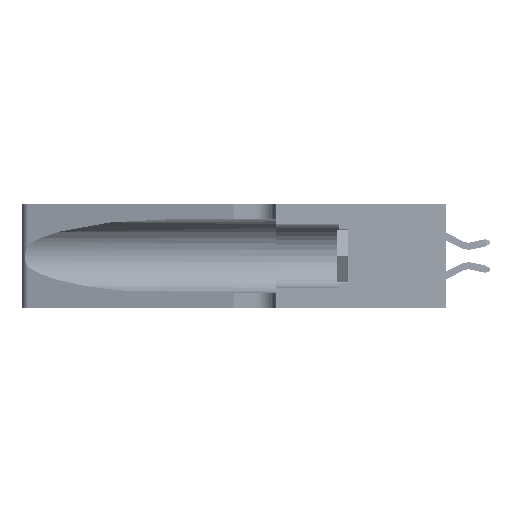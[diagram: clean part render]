
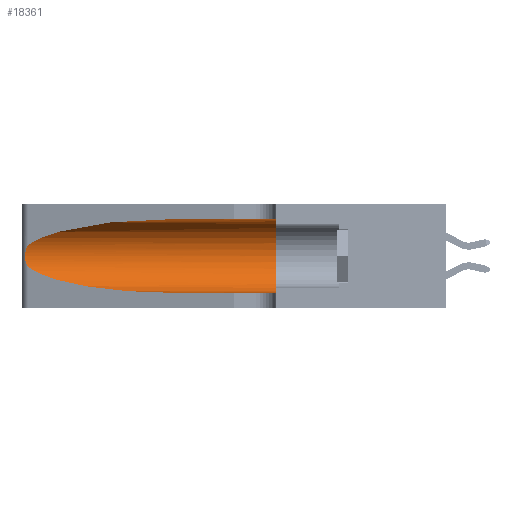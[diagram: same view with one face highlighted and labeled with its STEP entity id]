
A CAD part, left-side view. The second image highlights one B-rep face of the part: STEP entity #18361.
In plain terms, the highlighted cylindrical face has radius 3.308 mm (diameter 6.617 mm), a partial arc.
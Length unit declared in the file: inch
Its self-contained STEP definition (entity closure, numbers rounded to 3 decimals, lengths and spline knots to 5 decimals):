
#403 = ORIENTED_EDGE ( 'NONE', *, *, #45764, .T. ) ;
#1834 = CARTESIAN_POINT ( 'NONE',  ( 0.1305, 0.35, 0.05475 ) ) ;
#2414 = CARTESIAN_POINT ( 'NONE',  ( 0.25787, 1.23484, 0.2124 ) ) ;
#2507 = VERTEX_POINT ( 'NONE', #43651 ) ;
#5324 = FACE_OUTER_BOUND ( 'NONE', #14795, .T. ) ;
#5396 =( BOUNDED_CURVE ( )  B_SPLINE_CURVE ( 3, ( #17493, #8885, #21768, #51166 ),
 .UNSPECIFIED., .F., .F. ) 
 B_SPLINE_CURVE_WITH_KNOTS ( ( 4, 4 ),
 ( 3.44316, 4.71239 ),
 .UNSPECIFIED. ) 
 CURVE ( )  GEOMETRIC_REPRESENTATION_ITEM ( )  RATIONAL_B_SPLINE_CURVE ( ( 1., 0.87, 0.87, 1. ) ) 
 REPRESENTATION_ITEM ( '' )  );
#6060 = DIRECTION ( 'NONE',  ( 0., -1., 0. ) ) ;
#6214 = DIRECTION ( 'NONE',  ( 0., -1., 0. ) ) ;
#6706 = CARTESIAN_POINT ( 'NONE',  ( 0.26018, 1.23835, 0.19895 ) ) ;
#8131 = VERTEX_POINT ( 'NONE', #1834 ) ;
#8208 = EDGE_CURVE ( 'NONE', #21426, #42346, #44751, .T. ) ;
#8885 = CARTESIAN_POINT ( 'NONE',  ( 0.2373, 1.15595, 0.08982 ) ) ;
#11034 = CARTESIAN_POINT ( 'NONE',  ( 0.26075, 1.23896, 0.178 ) ) ;
#13370 = ORIENTED_EDGE ( 'NONE', *, *, #25348, .T. ) ;
#13740 = CARTESIAN_POINT ( 'NONE',  ( 0.1305, 0.35, 0.185 ) ) ;
#13960 = DIRECTION ( 'NONE',  ( 0., 0., -1. ) ) ;
#14795 = EDGE_LOOP ( 'NONE', ( #403, #54243, #37946, #13370, #43598, #37337 ) ) ;
#15139 = CARTESIAN_POINT ( 'NONE',  ( 0.25639, 1.23184, 0.21858 ) ) ;
#15327 = CARTESIAN_POINT ( 'NONE',  ( 0.25856, 1.23593, 0.16098 ) ) ;
#15800 = CARTESIAN_POINT ( 'NONE',  ( 0.1305, 0.72297, 0.05475 ) ) ;
#16131 = VECTOR ( 'NONE', #6060, 39.37008 ) ;
#16609 = CYLINDRICAL_SURFACE ( 'NONE', #29528, 0.13025 ) ;
#17493 = CARTESIAN_POINT ( 'NONE',  ( 0.25487, 1.22718, 0.14631 ) ) ;
#18043 = DIRECTION ( 'NONE',  ( 0., 0., 1. ) ) ;
#18361 = ADVANCED_FACE ( 'NONE', ( #5324 ), #16609, .F. ) ;
#18947 = CARTESIAN_POINT ( 'NONE',  ( 0.1305, 1.61858, 0.31525 ) ) ;
#19231 = CARTESIAN_POINT ( 'NONE',  ( 0.25487, 1.22718, 0.14631 ) ) ;
#19603 = CARTESIAN_POINT ( 'NONE',  ( 0.25639, 1.23186, 0.15144 ) ) ;
#19750 = CARTESIAN_POINT ( 'NONE',  ( 0.2373, 1.15595, 0.28018 ) ) ;
#20351 = LINE ( 'NONE', #35707, #52577 ) ;
#21426 = VERTEX_POINT ( 'NONE', #30051 ) ;
#21444 = EDGE_CURVE ( 'NONE', #42346, #41262, #5396, .T. ) ;
#21533 = CARTESIAN_POINT ( 'NONE',  ( 0.1305, 0.35, 0.31525 ) ) ;
#21768 = CARTESIAN_POINT ( 'NONE',  ( 0.18966, 0.96281, 0.05475 ) ) ;
#23408 = EDGE_CURVE ( 'NONE', #53689, #8131, #34042, .T. ) ;
#23883 = CARTESIAN_POINT ( 'NONE',  ( 0.25487, 1.22718, 0.14631 ) ) ;
#25348 = EDGE_CURVE ( 'NONE', #41262, #8131, #20351, .T. ) ;
#26603 = DIRECTION ( 'NONE',  ( 0., -1., 0. ) ) ;
#27412 = LINE ( 'NONE', #18947, #16131 ) ;
#27955 = CARTESIAN_POINT ( 'NONE',  ( 0.25487, 1.22718, 0.22369 ) ) ;
#28098 = CARTESIAN_POINT ( 'NONE',  ( 0.18966, 0.96281, 0.31525 ) ) ;
#29528 = AXIS2_PLACEMENT_3D ( 'NONE', #39287, #26603, #13960 ) ;
#30051 = CARTESIAN_POINT ( 'NONE',  ( 0.25487, 1.22718, 0.22369 ) ) ;
#32159 = CARTESIAN_POINT ( 'NONE',  ( 0.25854, 1.2359, 0.20912 ) ) ;
#34042 = CIRCLE ( 'NONE', #45827, 0.13025 ) ;
#35707 = CARTESIAN_POINT ( 'NONE',  ( 0.1305, 1.61858, 0.05475 ) ) ;
#36360 = CARTESIAN_POINT ( 'NONE',  ( 0.26075, 1.23896, 0.19203 ) ) ;
#36506 = CARTESIAN_POINT ( 'NONE',  ( 0.1305, 0.72297, 0.31525 ) ) ;
#36924 = EDGE_CURVE ( 'NONE', #2507, #53689, #27412, .T. ) ;
#37337 = ORIENTED_EDGE ( 'NONE', *, *, #36924, .F. ) ;
#37946 = ORIENTED_EDGE ( 'NONE', *, *, #21444, .T. ) ;
#39287 = CARTESIAN_POINT ( 'NONE',  ( 0.1305, 1.61858, 0.185 ) ) ;
#40603 = CARTESIAN_POINT ( 'NONE',  ( 0.26017, 1.23833, 0.17102 ) ) ;
#41262 = VERTEX_POINT ( 'NONE', #15800 ) ;
#42346 = VERTEX_POINT ( 'NONE', #19231 ) ;
#43267 = DIRECTION ( 'NONE',  ( 0., 1., 0. ) ) ;
#43598 = ORIENTED_EDGE ( 'NONE', *, *, #23408, .F. ) ;
#43651 = CARTESIAN_POINT ( 'NONE',  ( 0.1305, 0.72297, 0.31525 ) ) ;
#44751 = B_SPLINE_CURVE_WITH_KNOTS ( 'NONE', 3,
 ( #27955, #48854, #15139, #2414, #32159, #6706, #36360, #11034, #40603, #15327, #44808, #19603, #49036, #23883 ),
 .UNSPECIFIED., .F., .F.,
 ( 4, 2, 2, 2, 2, 2, 4 ),
 ( 0., 0.00027, 0.00053, 0.00107, 0.0016, 0.00187, 0.00214 ),
 .UNSPECIFIED. ) ;
#44808 = CARTESIAN_POINT ( 'NONE',  ( 0.25789, 1.23486, 0.15765 ) ) ;
#45764 = EDGE_CURVE ( 'NONE', #2507, #21426, #46415, .T. ) ;
#45827 = AXIS2_PLACEMENT_3D ( 'NONE', #13740, #43267, #18043 ) ;
#46415 =( BOUNDED_CURVE ( )  B_SPLINE_CURVE ( 3, ( #36506, #28098, #19750, #49187 ),
 .UNSPECIFIED., .F., .F. ) 
 B_SPLINE_CURVE_WITH_KNOTS ( ( 4, 4 ),
 ( 1.5708, 2.84003 ),
 .UNSPECIFIED. ) 
 CURVE ( )  GEOMETRIC_REPRESENTATION_ITEM ( )  RATIONAL_B_SPLINE_CURVE ( ( 1., 0.87, 0.87, 1. ) ) 
 REPRESENTATION_ITEM ( '' )  );
#48854 = CARTESIAN_POINT ( 'NONE',  ( 0.25555, 1.22994, 0.2215 ) ) ;
#49036 = CARTESIAN_POINT ( 'NONE',  ( 0.25555, 1.22993, 0.14849 ) ) ;
#49187 = CARTESIAN_POINT ( 'NONE',  ( 0.25487, 1.22718, 0.22369 ) ) ;
#51166 = CARTESIAN_POINT ( 'NONE',  ( 0.1305, 0.72297, 0.05475 ) ) ;
#52577 = VECTOR ( 'NONE', #6214, 39.37008 ) ;
#53689 = VERTEX_POINT ( 'NONE', #21533 ) ;
#54243 = ORIENTED_EDGE ( 'NONE', *, *, #8208, .T. ) ;
